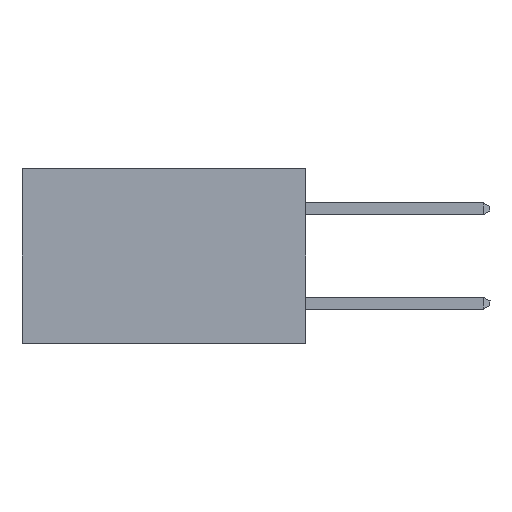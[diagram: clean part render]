
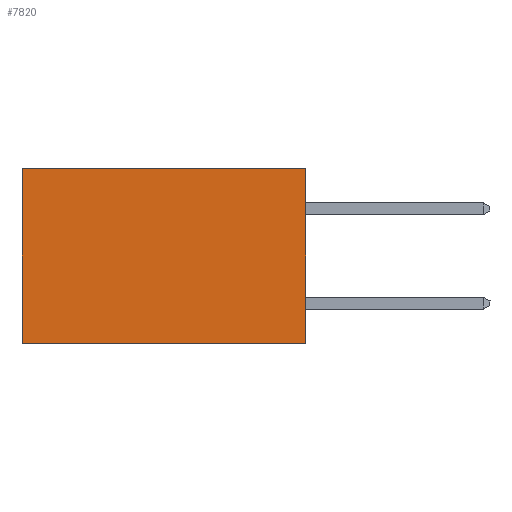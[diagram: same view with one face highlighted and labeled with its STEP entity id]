
A CAD part, left-side view. The second image highlights one B-rep face of the part: STEP entity #7820.
In plain terms, the highlighted planar face has unit normal (-1, 0, 0).
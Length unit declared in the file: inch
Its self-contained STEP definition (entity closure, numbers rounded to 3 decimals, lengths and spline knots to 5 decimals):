
#160 = VERTEX_POINT ( 'NONE', #10787 ) ;
#207 = DIRECTION ( 'NONE',  ( 1., 0., 0. ) ) ;
#714 = VECTOR ( 'NONE', #7359, 39.37008 ) ;
#1354 = CARTESIAN_POINT ( 'NONE',  ( 0.298, 0.6, 0. ) ) ;
#1528 = DIRECTION ( 'NONE',  ( 0., 1., 0. ) ) ;
#1783 = EDGE_CURVE ( 'NONE', #8320, #7805, #6645, .T. ) ;
#1888 = CARTESIAN_POINT ( 'NONE',  ( 0.298, 0., 0. ) ) ;
#1961 = ORIENTED_EDGE ( 'NONE', *, *, #8897, .T. ) ;
#2003 = VECTOR ( 'NONE', #2244, 39.37008 ) ;
#2244 = DIRECTION ( 'NONE',  ( 0., 0., -1. ) ) ;
#3197 = CARTESIAN_POINT ( 'NONE',  ( 0.298, 0.6, 0. ) ) ;
#3277 = ORIENTED_EDGE ( 'NONE', *, *, #3675, .F. ) ;
#3675 = EDGE_CURVE ( 'NONE', #160, #7805, #8941, .T. ) ;
#3691 = CARTESIAN_POINT ( 'NONE',  ( 0.298, 0.6, -0.37 ) ) ;
#3931 = CARTESIAN_POINT ( 'NONE',  ( 0.298, 0., 0. ) ) ;
#4093 = CARTESIAN_POINT ( 'NONE',  ( 0.298, 0., 0. ) ) ;
#4430 = PLANE ( 'NONE',  #10799 ) ;
#4573 = VECTOR ( 'NONE', #7344, 39.37008 ) ;
#4756 = VERTEX_POINT ( 'NONE', #4093 ) ;
#4777 = CARTESIAN_POINT ( 'NONE',  ( 0.298, 0., 0. ) ) ;
#5359 = VECTOR ( 'NONE', #1528, 39.37008 ) ;
#6508 = ORIENTED_EDGE ( 'NONE', *, *, #10775, .F. ) ;
#6645 = LINE ( 'NONE', #1354, #2003 ) ;
#6843 = LINE ( 'NONE', #4777, #4573 ) ;
#7344 = DIRECTION ( 'NONE',  ( 0., 0., -1. ) ) ;
#7359 = DIRECTION ( 'NONE',  ( 0., 1., 0. ) ) ;
#7632 = EDGE_LOOP ( 'NONE', ( #8410, #3277, #6508, #1961 ) ) ;
#7805 = VERTEX_POINT ( 'NONE', #3691 ) ;
#7820 = ADVANCED_FACE ( 'NONE', ( #10460 ), #4430, .F. ) ;
#7824 = DIRECTION ( 'NONE',  ( 0., 0., -1. ) ) ;
#8290 = CARTESIAN_POINT ( 'NONE',  ( 0.298, 0., -0.37 ) ) ;
#8320 = VERTEX_POINT ( 'NONE', #3197 ) ;
#8410 = ORIENTED_EDGE ( 'NONE', *, *, #1783, .T. ) ;
#8897 = EDGE_CURVE ( 'NONE', #4756, #8320, #9758, .T. ) ;
#8941 = LINE ( 'NONE', #8290, #5359 ) ;
#9758 = LINE ( 'NONE', #3931, #714 ) ;
#10460 = FACE_OUTER_BOUND ( 'NONE', #7632, .T. ) ;
#10775 = EDGE_CURVE ( 'NONE', #4756, #160, #6843, .T. ) ;
#10787 = CARTESIAN_POINT ( 'NONE',  ( 0.298, 0., -0.37 ) ) ;
#10799 = AXIS2_PLACEMENT_3D ( 'NONE', #1888, #207, #7824 ) ;
